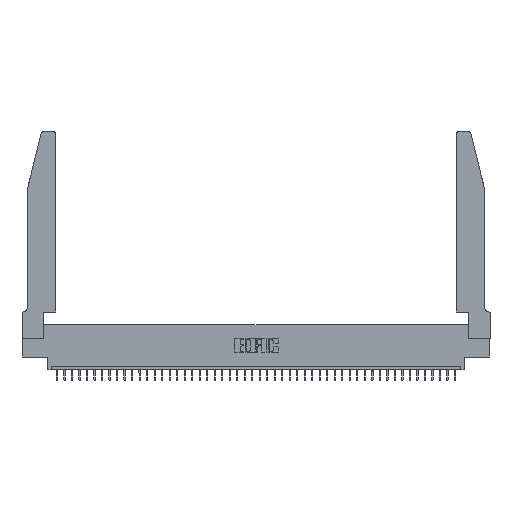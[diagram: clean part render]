
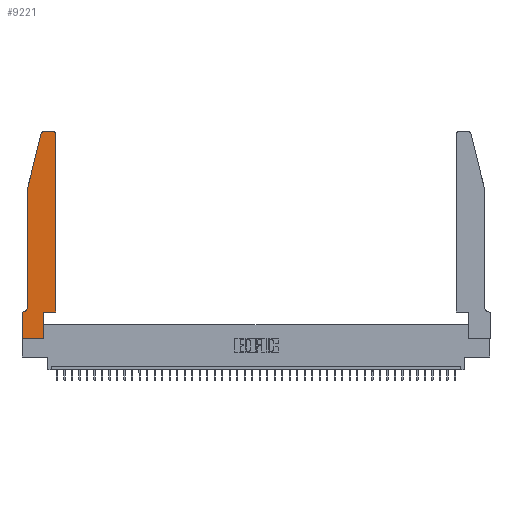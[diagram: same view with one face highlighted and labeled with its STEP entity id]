
A CAD part, top view. The second image highlights one B-rep face of the part: STEP entity #9221.
In plain terms, the highlighted planar face has unit normal (0, 0, 1).
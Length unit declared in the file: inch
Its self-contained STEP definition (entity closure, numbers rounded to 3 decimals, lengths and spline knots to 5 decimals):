
#59 = VERTEX_POINT ( 'NONE', #31259 ) ;
#351 = VERTEX_POINT ( 'NONE', #13891 ) ;
#720 = EDGE_CURVE ( 'NONE', #351, #17041, #19841, .T. ) ;
#1513 = CARTESIAN_POINT ( 'NONE',  ( 0., 0., 0.37 ) ) ;
#1694 = ORIENTED_EDGE ( 'NONE', *, *, #31160, .T. ) ;
#1753 = VERTEX_POINT ( 'NONE', #13670 ) ;
#1911 = EDGE_CURVE ( 'NONE', #17366, #59, #15906, .T. ) ;
#2623 = EDGE_CURVE ( 'NONE', #59, #30374, #23788, .T. ) ;
#2814 = EDGE_CURVE ( 'NONE', #20219, #16935, #39986, .T. ) ;
#2885 = VECTOR ( 'NONE', #20462, 39.37008 ) ;
#3379 = LINE ( 'NONE', #26292, #17463 ) ;
#4239 = ORIENTED_EDGE ( 'NONE', *, *, #34782, .T. ) ;
#4513 = CARTESIAN_POINT ( 'NONE',  ( 0.0055, 0.42, 0.37 ) ) ;
#5151 = VECTOR ( 'NONE', #13834, 39.37008 ) ;
#6038 = AXIS2_PLACEMENT_3D ( 'NONE', #42549, #15415, #28091 ) ;
#6269 = DIRECTION ( 'NONE',  ( -0.239, -0.971, 0. ) ) ;
#6774 = VERTEX_POINT ( 'NONE', #35194 ) ;
#6885 = CARTESIAN_POINT ( 'NONE',  ( 0.0755, 0.35, 0.37 ) ) ;
#8173 = CARTESIAN_POINT ( 'NONE',  ( 0.0755, 2., 0.37 ) ) ;
#8257 = AXIS2_PLACEMENT_3D ( 'NONE', #39397, #21595, #21823 ) ;
#8997 = CARTESIAN_POINT ( 'NONE',  ( 0.0755, 2., 0.37 ) ) ;
#9221 = ADVANCED_FACE ( 'NONE', ( #35826 ), #18710, .T. ) ;
#9319 = ORIENTED_EDGE ( 'NONE', *, *, #28696, .T. ) ;
#10005 = VECTOR ( 'NONE', #13059, 39.37008 ) ;
#10145 = CARTESIAN_POINT ( 'NONE',  ( 0.0755, 0.42, 0.37 ) ) ;
#10396 = VECTOR ( 'NONE', #26685, 39.37008 ) ;
#10504 = VECTOR ( 'NONE', #12122, 39.37008 ) ;
#12017 = AXIS2_PLACEMENT_3D ( 'NONE', #4513, #25850, #18089 ) ;
#12122 = DIRECTION ( 'NONE',  ( 0., -1., 0. ) ) ;
#13059 = DIRECTION ( 'NONE',  ( 1., 0., 0. ) ) ;
#13164 = CARTESIAN_POINT ( 'NONE',  ( 0.2865, 0.35, 0.37 ) ) ;
#13670 = CARTESIAN_POINT ( 'NONE',  ( 0.2865, 0.35, 0.37 ) ) ;
#13834 = DIRECTION ( 'NONE',  ( 0., 1., 0. ) ) ;
#13891 = CARTESIAN_POINT ( 'NONE',  ( 0.25487, 2.72718, 0.37 ) ) ;
#14302 = VERTEX_POINT ( 'NONE', #23094 ) ;
#14718 = CARTESIAN_POINT ( 'NONE',  ( 0.4205, 2.75, 0.37 ) ) ;
#15379 = CARTESIAN_POINT ( 'NONE',  ( 0., 0.35, 0.37 ) ) ;
#15415 = DIRECTION ( 'NONE',  ( 0., 0., 1. ) ) ;
#15906 = CIRCLE ( 'NONE', #12017, 0.07 ) ;
#16935 = VERTEX_POINT ( 'NONE', #20216 ) ;
#17041 = VERTEX_POINT ( 'NONE', #8173 ) ;
#17366 = VERTEX_POINT ( 'NONE', #10145 ) ;
#17463 = VECTOR ( 'NONE', #43438, 39.37008 ) ;
#18089 = DIRECTION ( 'NONE',  ( -1., 0., 0. ) ) ;
#18710 = PLANE ( 'NONE',  #32417 ) ;
#19616 = LINE ( 'NONE', #13164, #5151 ) ;
#19797 = LINE ( 'NONE', #40048, #10396 ) ;
#19841 = LINE ( 'NONE', #29624, #32869 ) ;
#20216 = CARTESIAN_POINT ( 'NONE',  ( 0.2865, 0., 0.37 ) ) ;
#20219 = VERTEX_POINT ( 'NONE', #1513 ) ;
#20462 = DIRECTION ( 'NONE',  ( -1., 0., 0. ) ) ;
#20490 = ORIENTED_EDGE ( 'NONE', *, *, #720, .T. ) ;
#20547 = ORIENTED_EDGE ( 'NONE', *, *, #25415, .T. ) ;
#21522 = LINE ( 'NONE', #35088, #24346 ) ;
#21595 = DIRECTION ( 'NONE',  ( 0., 0., 1. ) ) ;
#21823 = DIRECTION ( 'NONE',  ( 1., 0., 0. ) ) ;
#22254 = EDGE_CURVE ( 'NONE', #16935, #1753, #19616, .T. ) ;
#23094 = CARTESIAN_POINT ( 'NONE',  ( 0.4505, 2.72, 0.37 ) ) ;
#23788 = LINE ( 'NONE', #6885, #2885 ) ;
#24346 = VECTOR ( 'NONE', #28866, 39.37008 ) ;
#25231 = LINE ( 'NONE', #8997, #31005 ) ;
#25415 = EDGE_CURVE ( 'NONE', #14302, #34696, #26636, .T. ) ;
#25590 = DIRECTION ( 'NONE',  ( 1., 0., 0. ) ) ;
#25850 = DIRECTION ( 'NONE',  ( 0., 0., -1. ) ) ;
#26105 = DIRECTION ( 'NONE',  ( 0., -1., 0. ) ) ;
#26292 = CARTESIAN_POINT ( 'NONE',  ( 0.4505, 0.35, 0.37 ) ) ;
#26636 = CIRCLE ( 'NONE', #6038, 0.03 ) ;
#26685 = DIRECTION ( 'NONE',  ( -1., 0., 0. ) ) ;
#28091 = DIRECTION ( 'NONE',  ( 1., 0., 0. ) ) ;
#28514 = ORIENTED_EDGE ( 'NONE', *, *, #34399, .T. ) ;
#28598 = EDGE_CURVE ( 'NONE', #34696, #37657, #19797, .T. ) ;
#28696 = EDGE_CURVE ( 'NONE', #17041, #17366, #25231, .T. ) ;
#28866 = DIRECTION ( 'NONE',  ( 1., 0., 0. ) ) ;
#29086 = CARTESIAN_POINT ( 'NONE',  ( 0., 0., 0.37 ) ) ;
#29394 = CARTESIAN_POINT ( 'NONE',  ( 0., 0.35, 0.37 ) ) ;
#29624 = CARTESIAN_POINT ( 'NONE',  ( 0.0755, 2., 0.37 ) ) ;
#30238 = CARTESIAN_POINT ( 'NONE',  ( 0.284, 2.75, 0.37 ) ) ;
#30374 = VERTEX_POINT ( 'NONE', #29394 ) ;
#31005 = VECTOR ( 'NONE', #26105, 39.37008 ) ;
#31160 = EDGE_CURVE ( 'NONE', #1753, #6774, #21522, .T. ) ;
#31259 = CARTESIAN_POINT ( 'NONE',  ( 0.0055, 0.35, 0.37 ) ) ;
#31812 = EDGE_LOOP ( 'NONE', ( #36307, #4239, #20490, #9319, #42034, #32398, #43866, #39582, #34440, #1694, #28514, #20547 ) ) ;
#32398 = ORIENTED_EDGE ( 'NONE', *, *, #2623, .T. ) ;
#32417 = AXIS2_PLACEMENT_3D ( 'NONE', #15379, #32495, #25590 ) ;
#32495 = DIRECTION ( 'NONE',  ( 0., 0., 1. ) ) ;
#32798 = CARTESIAN_POINT ( 'NONE',  ( 0., 0., 0.37 ) ) ;
#32869 = VECTOR ( 'NONE', #6269, 39.37008 ) ;
#34399 = EDGE_CURVE ( 'NONE', #6774, #14302, #3379, .T. ) ;
#34440 = ORIENTED_EDGE ( 'NONE', *, *, #22254, .T. ) ;
#34696 = VERTEX_POINT ( 'NONE', #14718 ) ;
#34782 = EDGE_CURVE ( 'NONE', #37657, #351, #38117, .T. ) ;
#35088 = CARTESIAN_POINT ( 'NONE',  ( 0.4505, 0.35, 0.37 ) ) ;
#35194 = CARTESIAN_POINT ( 'NONE',  ( 0.4505, 0.35, 0.37 ) ) ;
#35826 = FACE_OUTER_BOUND ( 'NONE', #31812, .T. ) ;
#36307 = ORIENTED_EDGE ( 'NONE', *, *, #28598, .T. ) ;
#37657 = VERTEX_POINT ( 'NONE', #30238 ) ;
#38117 = CIRCLE ( 'NONE', #8257, 0.03 ) ;
#38523 = EDGE_CURVE ( 'NONE', #30374, #20219, #42611, .T. ) ;
#39397 = CARTESIAN_POINT ( 'NONE',  ( 0.284, 2.72, 0.37 ) ) ;
#39582 = ORIENTED_EDGE ( 'NONE', *, *, #2814, .T. ) ;
#39986 = LINE ( 'NONE', #29086, #10005 ) ;
#40048 = CARTESIAN_POINT ( 'NONE',  ( 0.2605, 2.75, 0.37 ) ) ;
#42034 = ORIENTED_EDGE ( 'NONE', *, *, #1911, .T. ) ;
#42549 = CARTESIAN_POINT ( 'NONE',  ( 0.4205, 2.72, 0.37 ) ) ;
#42611 = LINE ( 'NONE', #32798, #10504 ) ;
#43438 = DIRECTION ( 'NONE',  ( 0., 1., 0. ) ) ;
#43866 = ORIENTED_EDGE ( 'NONE', *, *, #38523, .T. ) ;
